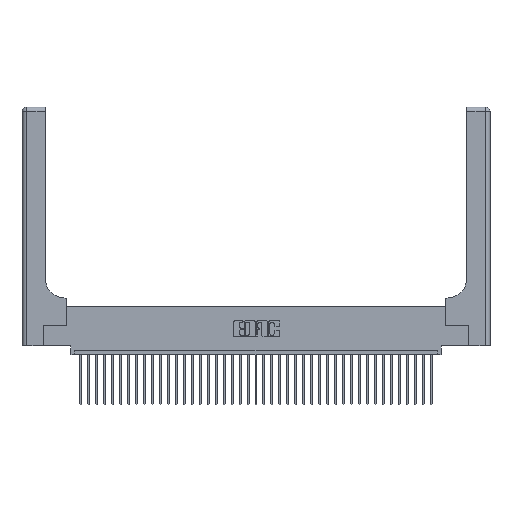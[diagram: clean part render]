
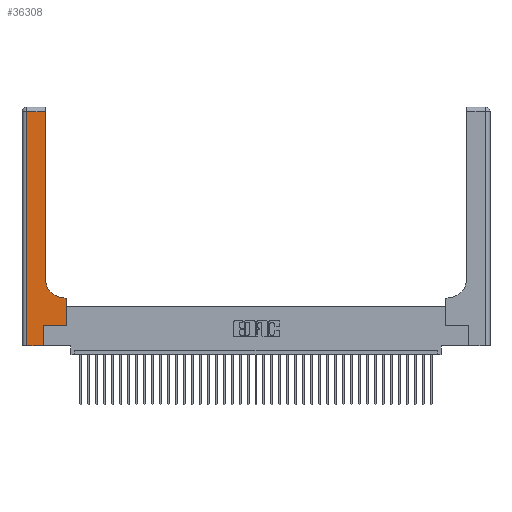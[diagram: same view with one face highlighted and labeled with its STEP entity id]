
A CAD part, top view. The second image highlights one B-rep face of the part: STEP entity #36308.
In plain terms, the highlighted planar face has unit normal (0, 0, 1).
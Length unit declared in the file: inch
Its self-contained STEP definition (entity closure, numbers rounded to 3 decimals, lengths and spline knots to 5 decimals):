
#392 = VERTEX_POINT ( 'NONE', #2075 ) ;
#1826 = AXIS2_PLACEMENT_3D ( 'NONE', #24323, #6417, #3697 ) ;
#1857 = DIRECTION ( 'NONE',  ( 1., 0., 0. ) ) ;
#2013 = VERTEX_POINT ( 'NONE', #2650 ) ;
#2075 = CARTESIAN_POINT ( 'NONE',  ( 0.269, 0., 0.37 ) ) ;
#2650 = CARTESIAN_POINT ( 'NONE',  ( 0.5585, 0.6, 0.37 ) ) ;
#3391 = ORIENTED_EDGE ( 'NONE', *, *, #21547, .T. ) ;
#3697 = DIRECTION ( 'NONE',  ( 1., 0., 0. ) ) ;
#4161 = CARTESIAN_POINT ( 'NONE',  ( 0.06, 0., 0.37 ) ) ;
#4236 = DIRECTION ( 'NONE',  ( 0., 1., 0. ) ) ;
#4237 = EDGE_CURVE ( 'NONE', #29740, #2013, #34267, .T. ) ;
#4425 = VECTOR ( 'NONE', #34531, 39.37008 ) ;
#4430 = LINE ( 'NONE', #19638, #31631 ) ;
#4849 = VERTEX_POINT ( 'NONE', #27698 ) ;
#5665 = CARTESIAN_POINT ( 'NONE',  ( 0., 2.94, 0.37 ) ) ;
#5987 = DIRECTION ( 'NONE',  ( 0., 0., -1. ) ) ;
#6417 = DIRECTION ( 'NONE',  ( 0., 0., -1. ) ) ;
#7177 = VERTEX_POINT ( 'NONE', #7867 ) ;
#7520 = VECTOR ( 'NONE', #9593, 39.37008 ) ;
#7598 = CARTESIAN_POINT ( 'NONE',  ( 0.269, 0.25, 0.37 ) ) ;
#7867 = CARTESIAN_POINT ( 'NONE',  ( 0.269, 0.25, 0.37 ) ) ;
#8168 = VECTOR ( 'NONE', #30676, 39.37008 ) ;
#8943 = EDGE_CURVE ( 'NONE', #4849, #36346, #37439, .T. ) ;
#9380 = ORIENTED_EDGE ( 'NONE', *, *, #26880, .T. ) ;
#9593 = DIRECTION ( 'NONE',  ( 0., 1., 0. ) ) ;
#11047 = CARTESIAN_POINT ( 'NONE',  ( 0.2915, 0.6, 0.37 ) ) ;
#12181 = ORIENTED_EDGE ( 'NONE', *, *, #4237, .T. ) ;
#13041 = VECTOR ( 'NONE', #16405, 39.37008 ) ;
#13652 = CARTESIAN_POINT ( 'NONE',  ( 0.2915, 0.85, 0.37 ) ) ;
#14553 = LINE ( 'NONE', #28811, #18708 ) ;
#14617 = ORIENTED_EDGE ( 'NONE', *, *, #16057, .T. ) ;
#14682 = DIRECTION ( 'NONE',  ( -1., 0., 0. ) ) ;
#15051 = CARTESIAN_POINT ( 'NONE',  ( 0.06, 2.94, 0.37 ) ) ;
#16057 = EDGE_CURVE ( 'NONE', #16752, #392, #4430, .T. ) ;
#16405 = DIRECTION ( 'NONE',  ( -1., 0., 0. ) ) ;
#16752 = VERTEX_POINT ( 'NONE', #4161 ) ;
#16961 = CARTESIAN_POINT ( 'NONE',  ( 0.5585, 0.25, 0.37 ) ) ;
#17719 = ORIENTED_EDGE ( 'NONE', *, *, #36755, .T. ) ;
#18261 = ORIENTED_EDGE ( 'NONE', *, *, #8943, .T. ) ;
#18460 = CARTESIAN_POINT ( 'NONE',  ( 0.5585, 0.25, 0.37 ) ) ;
#18570 = CARTESIAN_POINT ( 'NONE',  ( 0.06, 3., 0.37 ) ) ;
#18708 = VECTOR ( 'NONE', #34864, 39.37008 ) ;
#19638 = CARTESIAN_POINT ( 'NONE',  ( 0., 0., 0.37 ) ) ;
#20177 = AXIS2_PLACEMENT_3D ( 'NONE', #38514, #5987, #14682 ) ;
#20554 = EDGE_CURVE ( 'NONE', #7177, #29740, #21384, .T. ) ;
#21022 = DIRECTION ( 'NONE',  ( 1., 0., 0. ) ) ;
#21384 = LINE ( 'NONE', #7598, #37891 ) ;
#21547 = EDGE_CURVE ( 'NONE', #38619, #28962, #37152, .T. ) ;
#23025 = FACE_OUTER_BOUND ( 'NONE', #27913, .T. ) ;
#23171 = ORIENTED_EDGE ( 'NONE', *, *, #20554, .T. ) ;
#24020 = LINE ( 'NONE', #18570, #8168 ) ;
#24323 = CARTESIAN_POINT ( 'NONE',  ( 0.5415, 0.85, 0.37 ) ) ;
#25365 = ORIENTED_EDGE ( 'NONE', *, *, #28828, .T. ) ;
#26850 = LINE ( 'NONE', #11047, #4425 ) ;
#26880 = EDGE_CURVE ( 'NONE', #36346, #16752, #24020, .T. ) ;
#27069 = PLANE ( 'NONE',  #20177 ) ;
#27698 = CARTESIAN_POINT ( 'NONE',  ( 0.2915, 2.94, 0.37 ) ) ;
#27913 = EDGE_LOOP ( 'NONE', ( #25365, #18261, #9380, #14617, #17719, #23171, #12181, #27958, #3391 ) ) ;
#27958 = ORIENTED_EDGE ( 'NONE', *, *, #30211, .T. ) ;
#28811 = CARTESIAN_POINT ( 'NONE',  ( 0.269, 0., 0.37 ) ) ;
#28828 = EDGE_CURVE ( 'NONE', #28962, #4849, #32187, .T. ) ;
#28962 = VERTEX_POINT ( 'NONE', #13652 ) ;
#29740 = VERTEX_POINT ( 'NONE', #16961 ) ;
#30211 = EDGE_CURVE ( 'NONE', #2013, #38619, #26850, .T. ) ;
#30254 = CARTESIAN_POINT ( 'NONE',  ( 0.5415, 0.6, 0.37 ) ) ;
#30676 = DIRECTION ( 'NONE',  ( 0., -1., 0. ) ) ;
#31631 = VECTOR ( 'NONE', #1857, 39.37008 ) ;
#32187 = LINE ( 'NONE', #34527, #35015 ) ;
#34267 = LINE ( 'NONE', #18460, #7520 ) ;
#34527 = CARTESIAN_POINT ( 'NONE',  ( 0.2915, 3., 0.37 ) ) ;
#34531 = DIRECTION ( 'NONE',  ( -1., 0., 0. ) ) ;
#34864 = DIRECTION ( 'NONE',  ( 0., 1., 0. ) ) ;
#35015 = VECTOR ( 'NONE', #4236, 39.37008 ) ;
#36308 = ADVANCED_FACE ( 'NONE', ( #23025 ), #27069, .F. ) ;
#36346 = VERTEX_POINT ( 'NONE', #15051 ) ;
#36755 = EDGE_CURVE ( 'NONE', #392, #7177, #14553, .T. ) ;
#37152 = CIRCLE ( 'NONE', #1826, 0.25 ) ;
#37439 = LINE ( 'NONE', #5665, #13041 ) ;
#37891 = VECTOR ( 'NONE', #21022, 39.37008 ) ;
#38514 = CARTESIAN_POINT ( 'NONE',  ( 0., 3., 0.37 ) ) ;
#38619 = VERTEX_POINT ( 'NONE', #30254 ) ;
